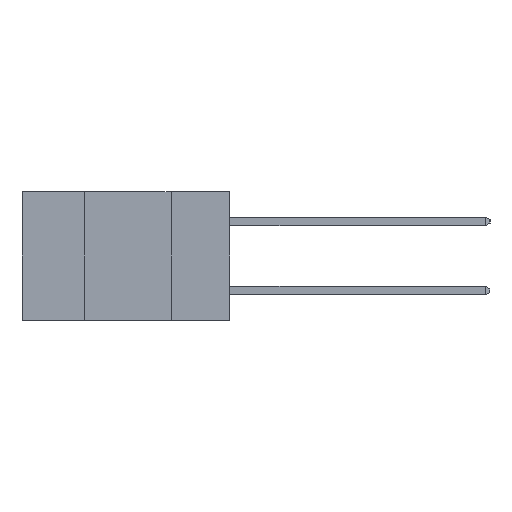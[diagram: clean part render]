
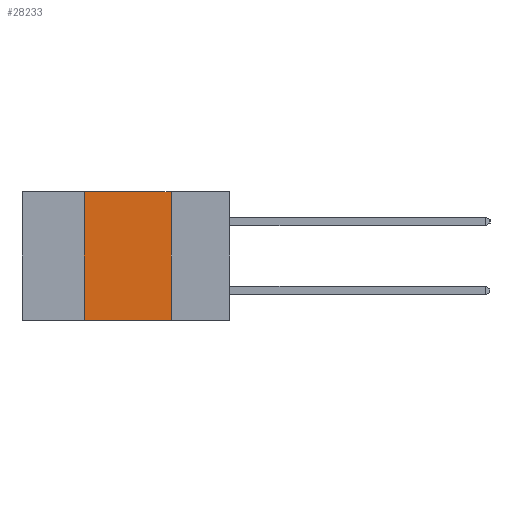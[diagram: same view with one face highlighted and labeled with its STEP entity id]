
A CAD part, left-side view. The second image highlights one B-rep face of the part: STEP entity #28233.
In plain terms, the highlighted planar face has unit normal (-1, 0, 0).
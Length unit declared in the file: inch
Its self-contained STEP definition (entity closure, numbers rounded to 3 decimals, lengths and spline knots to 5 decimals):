
#540 = EDGE_CURVE ( 'NONE', #1163, #13289, #21783, .T. ) ;
#737 = ORIENTED_EDGE ( 'NONE', *, *, #6033, .F. ) ;
#1163 = VERTEX_POINT ( 'NONE', #26676 ) ;
#3848 = CARTESIAN_POINT ( 'NONE',  ( 0., 0.6, -0.37 ) ) ;
#5888 = DIRECTION ( 'NONE',  ( 1., 0., 0. ) ) ;
#6033 = EDGE_CURVE ( 'NONE', #17914, #22859, #23939, .T. ) ;
#6043 = ORIENTED_EDGE ( 'NONE', *, *, #19169, .F. ) ;
#6324 = VECTOR ( 'NONE', #26808, 39.37008 ) ;
#6769 = AXIS2_PLACEMENT_3D ( 'NONE', #14963, #5888, #21813 ) ;
#8496 = EDGE_LOOP ( 'NONE', ( #22054, #6043, #737, #12843 ) ) ;
#9695 = VECTOR ( 'NONE', #17533, 39.37008 ) ;
#11696 = LINE ( 'NONE', #24564, #6324 ) ;
#11905 = VECTOR ( 'NONE', #28437, 39.37008 ) ;
#12843 = ORIENTED_EDGE ( 'NONE', *, *, #13862, .T. ) ;
#13289 = VERTEX_POINT ( 'NONE', #24834 ) ;
#13849 = CARTESIAN_POINT ( 'NONE',  ( 0., 0.42, -0.37 ) ) ;
#13862 = EDGE_CURVE ( 'NONE', #17914, #13289, #14470, .T. ) ;
#14470 = LINE ( 'NONE', #3848, #25791 ) ;
#14540 = CARTESIAN_POINT ( 'NONE',  ( 0., 0.17, 0. ) ) ;
#14963 = CARTESIAN_POINT ( 'NONE',  ( 0., 0.6, 0. ) ) ;
#17533 = DIRECTION ( 'NONE',  ( 0., 0., -1. ) ) ;
#17914 = VERTEX_POINT ( 'NONE', #13849 ) ;
#19169 = EDGE_CURVE ( 'NONE', #22859, #1163, #11696, .T. ) ;
#19336 = CARTESIAN_POINT ( 'NONE',  ( 0., 0.42, 0. ) ) ;
#21783 = LINE ( 'NONE', #14540, #9695 ) ;
#21813 = DIRECTION ( 'NONE',  ( 0., 0., -1. ) ) ;
#22054 = ORIENTED_EDGE ( 'NONE', *, *, #540, .F. ) ;
#22859 = VERTEX_POINT ( 'NONE', #25157 ) ;
#23939 = LINE ( 'NONE', #19336, #11905 ) ;
#23977 = PLANE ( 'NONE',  #6769 ) ;
#24308 = DIRECTION ( 'NONE',  ( 0., -1., 0. ) ) ;
#24564 = CARTESIAN_POINT ( 'NONE',  ( 0., 0.6, 0. ) ) ;
#24834 = CARTESIAN_POINT ( 'NONE',  ( 0., 0.17, -0.37 ) ) ;
#25157 = CARTESIAN_POINT ( 'NONE',  ( 0., 0.42, 0. ) ) ;
#25791 = VECTOR ( 'NONE', #24308, 39.37008 ) ;
#26676 = CARTESIAN_POINT ( 'NONE',  ( 0., 0.17, 0. ) ) ;
#26808 = DIRECTION ( 'NONE',  ( 0., -1., 0. ) ) ;
#27839 = FACE_OUTER_BOUND ( 'NONE', #8496, .T. ) ;
#28233 = ADVANCED_FACE ( 'NONE', ( #27839 ), #23977, .F. ) ;
#28437 = DIRECTION ( 'NONE',  ( 0., 0., 1. ) ) ;
